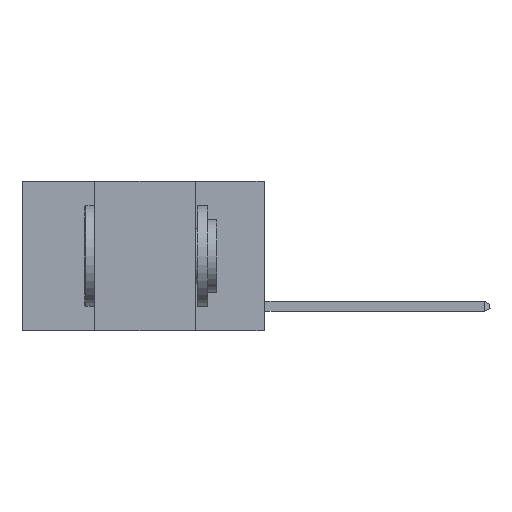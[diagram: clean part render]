
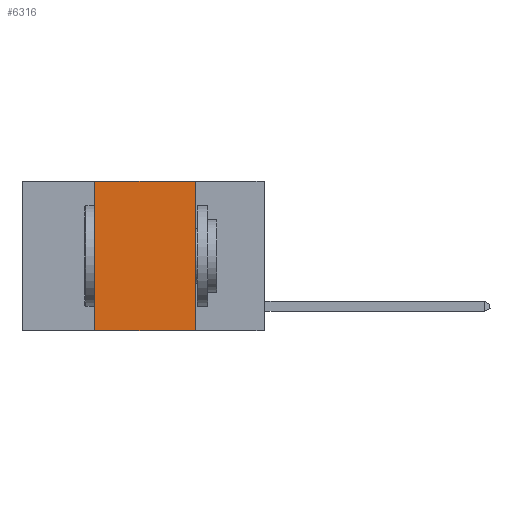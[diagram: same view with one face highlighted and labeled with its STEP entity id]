
A CAD part, left-side view. The second image highlights one B-rep face of the part: STEP entity #6316.
In plain terms, the highlighted planar face has unit normal (-1, 0, 0).
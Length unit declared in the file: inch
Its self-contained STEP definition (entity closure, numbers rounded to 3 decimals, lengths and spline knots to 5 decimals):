
#631 = VECTOR ( 'NONE', #13144, 39.37008 ) ;
#905 = CARTESIAN_POINT ( 'NONE',  ( 0., 0.17, -0.37 ) ) ;
#982 = EDGE_CURVE ( 'NONE', #10237, #5391, #21775, .T. ) ;
#1014 = VECTOR ( 'NONE', #21084, 39.37008 ) ;
#1187 = FACE_OUTER_BOUND ( 'NONE', #1268, .T. ) ;
#1268 = EDGE_LOOP ( 'NONE', ( #12750, #17207, #2754, #7322 ) ) ;
#1410 = DIRECTION ( 'NONE',  ( 0., 0., -1. ) ) ;
#1652 = LINE ( 'NONE', #10408, #13203 ) ;
#2362 = DIRECTION ( 'NONE',  ( 0., 0., -1. ) ) ;
#2629 = CARTESIAN_POINT ( 'NONE',  ( 0., 0.17, 0. ) ) ;
#2754 = ORIENTED_EDGE ( 'NONE', *, *, #982, .F. ) ;
#3501 = EDGE_CURVE ( 'NONE', #5391, #10737, #1652, .T. ) ;
#3791 = VECTOR ( 'NONE', #2362, 39.37008 ) ;
#4408 = CARTESIAN_POINT ( 'NONE',  ( 0., 0.42, -0.37 ) ) ;
#4897 = EDGE_CURVE ( 'NONE', #10237, #15437, #13933, .T. ) ;
#5038 = PLANE ( 'NONE',  #16320 ) ;
#5391 = VERTEX_POINT ( 'NONE', #18520 ) ;
#6197 = CARTESIAN_POINT ( 'NONE',  ( 0., 0.42, 0. ) ) ;
#6316 = ADVANCED_FACE ( 'NONE', ( #1187 ), #5038, .F. ) ;
#7322 = ORIENTED_EDGE ( 'NONE', *, *, #4897, .T. ) ;
#9411 = LINE ( 'NONE', #16109, #3791 ) ;
#10237 = VERTEX_POINT ( 'NONE', #4408 ) ;
#10408 = CARTESIAN_POINT ( 'NONE',  ( 0., 0.6, 0. ) ) ;
#10737 = VERTEX_POINT ( 'NONE', #2629 ) ;
#11182 = DIRECTION ( 'NONE',  ( 0., -1., 0. ) ) ;
#12750 = ORIENTED_EDGE ( 'NONE', *, *, #21479, .F. ) ;
#13144 = DIRECTION ( 'NONE',  ( 0., 0., 1. ) ) ;
#13203 = VECTOR ( 'NONE', #11182, 39.37008 ) ;
#13933 = LINE ( 'NONE', #20860, #1014 ) ;
#15437 = VERTEX_POINT ( 'NONE', #905 ) ;
#16109 = CARTESIAN_POINT ( 'NONE',  ( 0., 0.17, 0. ) ) ;
#16320 = AXIS2_PLACEMENT_3D ( 'NONE', #18577, #16855, #1410 ) ;
#16855 = DIRECTION ( 'NONE',  ( 1., 0., 0. ) ) ;
#17207 = ORIENTED_EDGE ( 'NONE', *, *, #3501, .F. ) ;
#18520 = CARTESIAN_POINT ( 'NONE',  ( 0., 0.42, 0. ) ) ;
#18577 = CARTESIAN_POINT ( 'NONE',  ( 0., 0.6, 0. ) ) ;
#20860 = CARTESIAN_POINT ( 'NONE',  ( 0., 0.6, -0.37 ) ) ;
#21084 = DIRECTION ( 'NONE',  ( 0., -1., 0. ) ) ;
#21479 = EDGE_CURVE ( 'NONE', #10737, #15437, #9411, .T. ) ;
#21775 = LINE ( 'NONE', #6197, #631 ) ;
